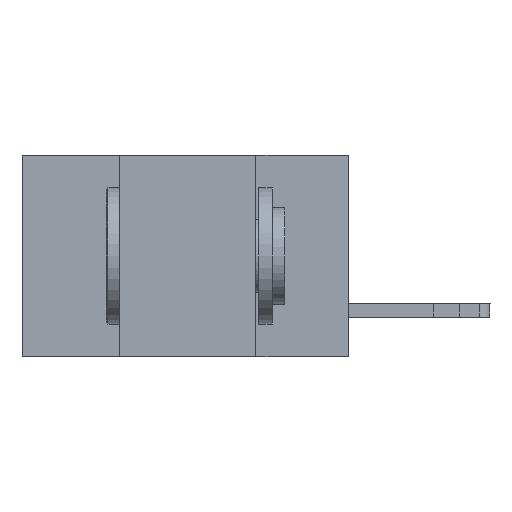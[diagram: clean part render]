
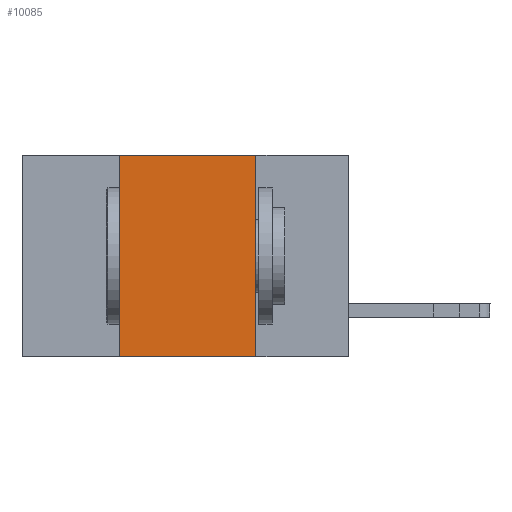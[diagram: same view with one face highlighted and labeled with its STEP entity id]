
A CAD part, left-side view. The second image highlights one B-rep face of the part: STEP entity #10085.
In plain terms, the highlighted planar face has unit normal (-1, 0, 0).
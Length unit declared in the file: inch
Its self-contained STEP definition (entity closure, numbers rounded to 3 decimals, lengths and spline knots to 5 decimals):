
#360 = ORIENTED_EDGE ( 'NONE', *, *, #11204, .F. ) ;
#471 = VERTEX_POINT ( 'NONE', #9220 ) ;
#944 = ORIENTED_EDGE ( 'NONE', *, *, #9377, .T. ) ;
#1289 = LINE ( 'NONE', #11259, #1636 ) ;
#1435 = EDGE_LOOP ( 'NONE', ( #7623, #9436, #360, #944 ) ) ;
#1564 = VERTEX_POINT ( 'NONE', #8866 ) ;
#1636 = VECTOR ( 'NONE', #4909, 39.37008 ) ;
#2731 = VERTEX_POINT ( 'NONE', #6444 ) ;
#3164 = VECTOR ( 'NONE', #4588, 39.37008 ) ;
#3398 = CARTESIAN_POINT ( 'NONE',  ( 0., 0.6, 0. ) ) ;
#3730 = EDGE_CURVE ( 'NONE', #471, #1564, #1289, .T. ) ;
#3782 = DIRECTION ( 'NONE',  ( 0., -1., 0. ) ) ;
#4098 = LINE ( 'NONE', #11464, #5501 ) ;
#4295 = FACE_OUTER_BOUND ( 'NONE', #1435, .T. ) ;
#4588 = DIRECTION ( 'NONE',  ( 0., 0., 1. ) ) ;
#4909 = DIRECTION ( 'NONE',  ( 0., -1., 0. ) ) ;
#5340 = VECTOR ( 'NONE', #3782, 39.37008 ) ;
#5501 = VECTOR ( 'NONE', #6678, 39.37008 ) ;
#5624 = LINE ( 'NONE', #11150, #5340 ) ;
#6020 = DIRECTION ( 'NONE',  ( 0., 0., -1. ) ) ;
#6088 = VERTEX_POINT ( 'NONE', #6932 ) ;
#6373 = LINE ( 'NONE', #10209, #3164 ) ;
#6444 = CARTESIAN_POINT ( 'NONE',  ( 0., 0.17, -0.37 ) ) ;
#6678 = DIRECTION ( 'NONE',  ( 0., 0., -1. ) ) ;
#6932 = CARTESIAN_POINT ( 'NONE',  ( 0., 0.42, -0.37 ) ) ;
#7127 = DIRECTION ( 'NONE',  ( 1., 0., 0. ) ) ;
#7450 = EDGE_CURVE ( 'NONE', #1564, #2731, #4098, .T. ) ;
#7623 = ORIENTED_EDGE ( 'NONE', *, *, #7450, .F. ) ;
#8866 = CARTESIAN_POINT ( 'NONE',  ( 0., 0.17, 0. ) ) ;
#9220 = CARTESIAN_POINT ( 'NONE',  ( 0., 0.42, 0. ) ) ;
#9377 = EDGE_CURVE ( 'NONE', #6088, #2731, #5624, .T. ) ;
#9436 = ORIENTED_EDGE ( 'NONE', *, *, #3730, .F. ) ;
#10085 = ADVANCED_FACE ( 'NONE', ( #4295 ), #10706, .F. ) ;
#10209 = CARTESIAN_POINT ( 'NONE',  ( 0., 0.42, -0.37 ) ) ;
#10706 = PLANE ( 'NONE',  #11627 ) ;
#11150 = CARTESIAN_POINT ( 'NONE',  ( 0., 0.6, -0.37 ) ) ;
#11204 = EDGE_CURVE ( 'NONE', #6088, #471, #6373, .T. ) ;
#11259 = CARTESIAN_POINT ( 'NONE',  ( 0., 0.6, 0. ) ) ;
#11464 = CARTESIAN_POINT ( 'NONE',  ( 0., 0.17, -0.37 ) ) ;
#11627 = AXIS2_PLACEMENT_3D ( 'NONE', #3398, #7127, #6020 ) ;
